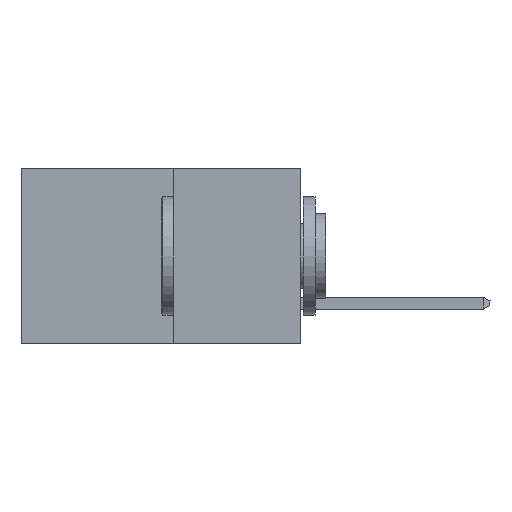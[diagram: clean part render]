
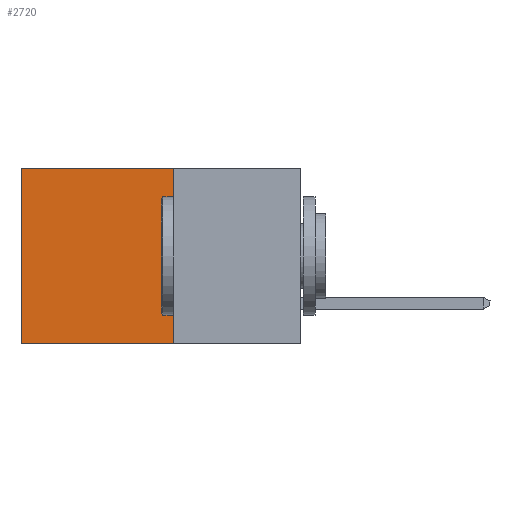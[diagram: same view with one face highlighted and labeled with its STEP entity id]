
A CAD part, left-side view. The second image highlights one B-rep face of the part: STEP entity #2720.
In plain terms, the highlighted planar face has unit normal (-1, 0, 0).
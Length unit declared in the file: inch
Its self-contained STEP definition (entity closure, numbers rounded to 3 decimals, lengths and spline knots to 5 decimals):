
#5 = VERTEX_POINT ( 'NONE', #12036 ) ;
#321 = LINE ( 'NONE', #5140, #8669 ) ;
#483 = CARTESIAN_POINT ( 'NONE',  ( 0.277, 0.27, -0.37 ) ) ;
#612 = CARTESIAN_POINT ( 'NONE',  ( 0.277, 0.59, -0.37 ) ) ;
#1458 = VERTEX_POINT ( 'NONE', #5210 ) ;
#1553 = DIRECTION ( 'NONE',  ( 1., 0., 0. ) ) ;
#1934 = LINE ( 'NONE', #612, #4477 ) ;
#2720 = ADVANCED_FACE ( 'NONE', ( #6645 ), #3607, .F. ) ;
#2736 = VERTEX_POINT ( 'NONE', #11151 ) ;
#3211 = CARTESIAN_POINT ( 'NONE',  ( 0.277, 0.27, -0.37 ) ) ;
#3287 = AXIS2_PLACEMENT_3D ( 'NONE', #483, #1553, #12381 ) ;
#3607 = PLANE ( 'NONE',  #3287 ) ;
#4088 = ORIENTED_EDGE ( 'NONE', *, *, #11735, .T. ) ;
#4164 = LINE ( 'NONE', #3211, #4488 ) ;
#4477 = VECTOR ( 'NONE', #13581, 39.37008 ) ;
#4488 = VECTOR ( 'NONE', #13946, 39.37008 ) ;
#5140 = CARTESIAN_POINT ( 'NONE',  ( 0.277, 0.27, -0.37 ) ) ;
#5210 = CARTESIAN_POINT ( 'NONE',  ( 0.277, 0.59, 0. ) ) ;
#6208 = DIRECTION ( 'NONE',  ( 0., 1., 0. ) ) ;
#6262 = CARTESIAN_POINT ( 'NONE',  ( 0.277, 0.27, 0. ) ) ;
#6401 = VERTEX_POINT ( 'NONE', #9926 ) ;
#6645 = FACE_OUTER_BOUND ( 'NONE', #8069, .T. ) ;
#7287 = LINE ( 'NONE', #6262, #13352 ) ;
#8069 = EDGE_LOOP ( 'NONE', ( #10130, #12638, #9791, #4088 ) ) ;
#8394 = DIRECTION ( 'NONE',  ( 0., 1., 0. ) ) ;
#8626 = EDGE_CURVE ( 'NONE', #2736, #6401, #321, .T. ) ;
#8669 = VECTOR ( 'NONE', #6208, 39.37008 ) ;
#8765 = EDGE_CURVE ( 'NONE', #5, #2736, #4164, .T. ) ;
#9181 = EDGE_CURVE ( 'NONE', #1458, #6401, #1934, .T. ) ;
#9791 = ORIENTED_EDGE ( 'NONE', *, *, #8765, .F. ) ;
#9926 = CARTESIAN_POINT ( 'NONE',  ( 0.277, 0.59, -0.37 ) ) ;
#10130 = ORIENTED_EDGE ( 'NONE', *, *, #9181, .T. ) ;
#11151 = CARTESIAN_POINT ( 'NONE',  ( 0.277, 0.27, -0.37 ) ) ;
#11735 = EDGE_CURVE ( 'NONE', #5, #1458, #7287, .T. ) ;
#12036 = CARTESIAN_POINT ( 'NONE',  ( 0.277, 0.27, 0. ) ) ;
#12381 = DIRECTION ( 'NONE',  ( 0., 0., -1. ) ) ;
#12638 = ORIENTED_EDGE ( 'NONE', *, *, #8626, .F. ) ;
#13352 = VECTOR ( 'NONE', #8394, 39.37008 ) ;
#13581 = DIRECTION ( 'NONE',  ( 0., 0., -1. ) ) ;
#13946 = DIRECTION ( 'NONE',  ( 0., 0., -1. ) ) ;
